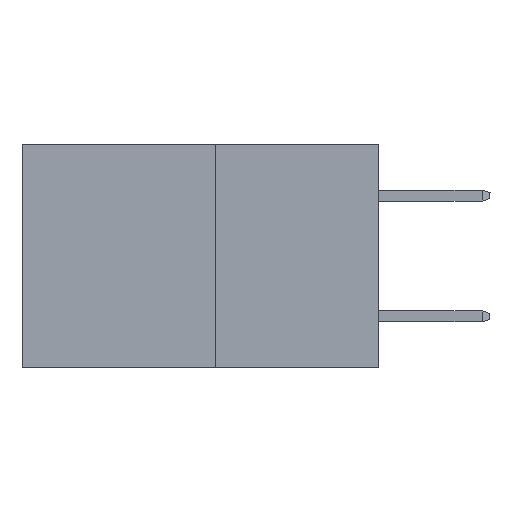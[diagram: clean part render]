
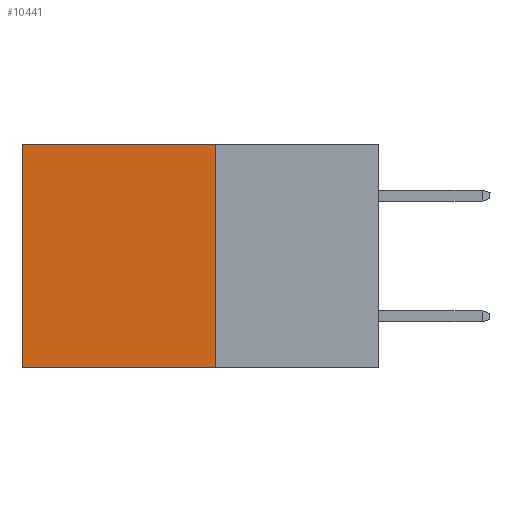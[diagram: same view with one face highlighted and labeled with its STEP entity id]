
A CAD part, left-side view. The second image highlights one B-rep face of the part: STEP entity #10441.
In plain terms, the highlighted planar face has unit normal (-1, 0, 0).
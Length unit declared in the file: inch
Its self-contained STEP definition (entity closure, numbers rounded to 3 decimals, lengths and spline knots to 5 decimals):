
#117 = DIRECTION ( 'NONE',  ( 0., 1., 0. ) ) ;
#404 = CARTESIAN_POINT ( 'NONE',  ( 0.277, 0.27, -0.37 ) ) ;
#551 = CARTESIAN_POINT ( 'NONE',  ( 0.277, 0.27, -0.37 ) ) ;
#1149 = VERTEX_POINT ( 'NONE', #7963 ) ;
#1151 = DIRECTION ( 'NONE',  ( 0., 0., -1. ) ) ;
#1299 = CARTESIAN_POINT ( 'NONE',  ( 0.277, 0.59, -0.37 ) ) ;
#1538 = EDGE_CURVE ( 'NONE', #11091, #3099, #10306, .T. ) ;
#1634 = CARTESIAN_POINT ( 'NONE',  ( 0.277, 0.59, -0.37 ) ) ;
#2512 = DIRECTION ( 'NONE',  ( 0., 0., -1. ) ) ;
#2600 = FACE_OUTER_BOUND ( 'NONE', #3452, .T. ) ;
#2692 = CARTESIAN_POINT ( 'NONE',  ( 0.277, 0.27, 0. ) ) ;
#2774 = DIRECTION ( 'NONE',  ( 0., 0., -1. ) ) ;
#3099 = VERTEX_POINT ( 'NONE', #404 ) ;
#3449 = VECTOR ( 'NONE', #2774, 39.37008 ) ;
#3452 = EDGE_LOOP ( 'NONE', ( #5555, #10080, #3485, #5821 ) ) ;
#3485 = ORIENTED_EDGE ( 'NONE', *, *, #1538, .F. ) ;
#3759 = VERTEX_POINT ( 'NONE', #1299 ) ;
#3977 = EDGE_CURVE ( 'NONE', #3099, #3759, #4013, .T. ) ;
#4013 = LINE ( 'NONE', #7722, #10578 ) ;
#4273 = AXIS2_PLACEMENT_3D ( 'NONE', #5549, #6406, #1151 ) ;
#4674 = PLANE ( 'NONE',  #4273 ) ;
#5366 = VECTOR ( 'NONE', #2512, 39.37008 ) ;
#5549 = CARTESIAN_POINT ( 'NONE',  ( 0.277, 0.27, -0.37 ) ) ;
#5555 = ORIENTED_EDGE ( 'NONE', *, *, #10143, .T. ) ;
#5600 = EDGE_CURVE ( 'NONE', #11091, #1149, #6430, .T. ) ;
#5821 = ORIENTED_EDGE ( 'NONE', *, *, #5600, .T. ) ;
#6167 = VECTOR ( 'NONE', #117, 39.37008 ) ;
#6321 = CARTESIAN_POINT ( 'NONE',  ( 0.277, 0.27, 0. ) ) ;
#6406 = DIRECTION ( 'NONE',  ( 1., 0., 0. ) ) ;
#6430 = LINE ( 'NONE', #6321, #6167 ) ;
#7663 = LINE ( 'NONE', #1634, #5366 ) ;
#7722 = CARTESIAN_POINT ( 'NONE',  ( 0.277, 0.27, -0.37 ) ) ;
#7963 = CARTESIAN_POINT ( 'NONE',  ( 0.277, 0.59, 0. ) ) ;
#8562 = DIRECTION ( 'NONE',  ( 0., 1., 0. ) ) ;
#10080 = ORIENTED_EDGE ( 'NONE', *, *, #3977, .F. ) ;
#10143 = EDGE_CURVE ( 'NONE', #1149, #3759, #7663, .T. ) ;
#10306 = LINE ( 'NONE', #551, #3449 ) ;
#10441 = ADVANCED_FACE ( 'NONE', ( #2600 ), #4674, .F. ) ;
#10578 = VECTOR ( 'NONE', #8562, 39.37008 ) ;
#11091 = VERTEX_POINT ( 'NONE', #2692 ) ;
